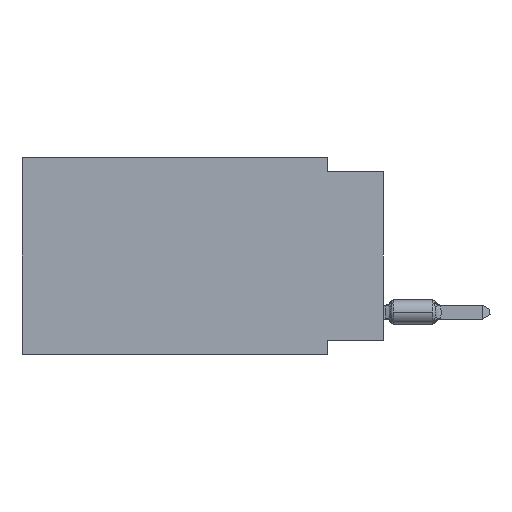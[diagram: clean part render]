
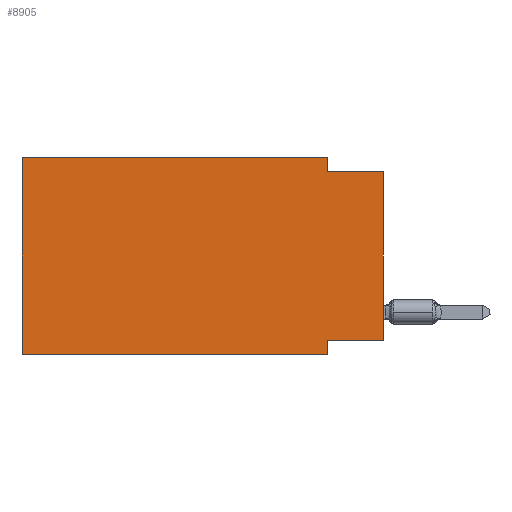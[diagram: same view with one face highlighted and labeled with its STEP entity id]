
A CAD part, left-side view. The second image highlights one B-rep face of the part: STEP entity #8905.
In plain terms, the highlighted planar face has unit normal (-1, 0, 0).
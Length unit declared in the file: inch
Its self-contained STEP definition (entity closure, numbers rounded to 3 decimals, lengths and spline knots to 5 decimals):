
#45 = ORIENTED_EDGE ( 'NONE', *, *, #11545, .F. ) ;
#162 = CARTESIAN_POINT ( 'NONE',  ( 0., 0.645, -0.35 ) ) ;
#1370 = EDGE_CURVE ( 'NONE', #24285, #9462, #19959, .T. ) ;
#2396 = CARTESIAN_POINT ( 'NONE',  ( 0., 0.645, 0. ) ) ;
#3505 = CARTESIAN_POINT ( 'NONE',  ( 0., 0., -0.025 ) ) ;
#4246 = CARTESIAN_POINT ( 'NONE',  ( 0., 0., 0. ) ) ;
#4253 = CARTESIAN_POINT ( 'NONE',  ( 0., 0.1, -0.35 ) ) ;
#4673 = VECTOR ( 'NONE', #25374, 39.37008 ) ;
#6394 = VERTEX_POINT ( 'NONE', #11182 ) ;
#8007 = ORIENTED_EDGE ( 'NONE', *, *, #1370, .T. ) ;
#8520 = LINE ( 'NONE', #3505, #23439 ) ;
#8905 = ADVANCED_FACE ( 'NONE', ( #8964 ), #26022, .F. ) ;
#8964 = FACE_OUTER_BOUND ( 'NONE', #26578, .T. ) ;
#9452 = DIRECTION ( 'NONE',  ( 0., 0., -1. ) ) ;
#9462 = VERTEX_POINT ( 'NONE', #4253 ) ;
#10016 = ORIENTED_EDGE ( 'NONE', *, *, #18518, .T. ) ;
#10137 = VECTOR ( 'NONE', #22067, 39.37008 ) ;
#11182 = CARTESIAN_POINT ( 'NONE',  ( 0., 0., -0.025 ) ) ;
#11545 = EDGE_CURVE ( 'NONE', #32569, #17454, #35048, .T. ) ;
#12277 = AXIS2_PLACEMENT_3D ( 'NONE', #20252, #34721, #31595 ) ;
#13500 = LINE ( 'NONE', #2396, #34774 ) ;
#14606 = ORIENTED_EDGE ( 'NONE', *, *, #29469, .F. ) ;
#15183 = ORIENTED_EDGE ( 'NONE', *, *, #36416, .F. ) ;
#15213 = VERTEX_POINT ( 'NONE', #34568 ) ;
#16543 = CARTESIAN_POINT ( 'NONE',  ( 0., 0.645, -0.35 ) ) ;
#16590 = LINE ( 'NONE', #22883, #17848 ) ;
#17033 = VERTEX_POINT ( 'NONE', #29630 ) ;
#17454 = VERTEX_POINT ( 'NONE', #18063 ) ;
#17838 = ORIENTED_EDGE ( 'NONE', *, *, #32672, .F. ) ;
#17848 = VECTOR ( 'NONE', #36665, 39.37008 ) ;
#18063 = CARTESIAN_POINT ( 'NONE',  ( 0., 0.1, -0.025 ) ) ;
#18518 = EDGE_CURVE ( 'NONE', #17033, #6394, #19054, .T. ) ;
#19054 = LINE ( 'NONE', #4246, #22091 ) ;
#19959 = LINE ( 'NONE', #162, #4673 ) ;
#20252 = CARTESIAN_POINT ( 'NONE',  ( 0., 0.645, 0. ) ) ;
#20347 = DIRECTION ( 'NONE',  ( 0., -1., 0. ) ) ;
#21973 = VECTOR ( 'NONE', #9452, 39.37008 ) ;
#22067 = DIRECTION ( 'NONE',  ( 0., 0., 1. ) ) ;
#22091 = VECTOR ( 'NONE', #29824, 39.37008 ) ;
#22205 = DIRECTION ( 'NONE',  ( 0., -1., 0. ) ) ;
#22883 = CARTESIAN_POINT ( 'NONE',  ( 0., 0., -0.325 ) ) ;
#22989 = VECTOR ( 'NONE', #27749, 39.37008 ) ;
#23093 = EDGE_CURVE ( 'NONE', #15213, #32569, #13500, .T. ) ;
#23439 = VECTOR ( 'NONE', #20347, 39.37008 ) ;
#23898 = CARTESIAN_POINT ( 'NONE',  ( 0., 0.1, 0. ) ) ;
#24285 = VERTEX_POINT ( 'NONE', #16543 ) ;
#24660 = CARTESIAN_POINT ( 'NONE',  ( 0., 0.645, 0. ) ) ;
#25374 = DIRECTION ( 'NONE',  ( 0., -1., 0. ) ) ;
#26022 = PLANE ( 'NONE',  #12277 ) ;
#26578 = EDGE_LOOP ( 'NONE', ( #10016, #17838, #45, #35290, #33995, #8007, #15183, #14606 ) ) ;
#27449 = EDGE_CURVE ( 'NONE', #24285, #15213, #36382, .T. ) ;
#27749 = DIRECTION ( 'NONE',  ( 0., 0., -1. ) ) ;
#28303 = LINE ( 'NONE', #36297, #22989 ) ;
#29469 = EDGE_CURVE ( 'NONE', #17033, #29840, #16590, .T. ) ;
#29630 = CARTESIAN_POINT ( 'NONE',  ( 0., 0., -0.325 ) ) ;
#29824 = DIRECTION ( 'NONE',  ( 0., 0., 1. ) ) ;
#29840 = VERTEX_POINT ( 'NONE', #35145 ) ;
#31595 = DIRECTION ( 'NONE',  ( 0., 0., -1. ) ) ;
#32569 = VERTEX_POINT ( 'NONE', #35982 ) ;
#32672 = EDGE_CURVE ( 'NONE', #17454, #6394, #8520, .T. ) ;
#33995 = ORIENTED_EDGE ( 'NONE', *, *, #27449, .F. ) ;
#34568 = CARTESIAN_POINT ( 'NONE',  ( 0., 0.645, 0. ) ) ;
#34721 = DIRECTION ( 'NONE',  ( 1., 0., 0. ) ) ;
#34774 = VECTOR ( 'NONE', #22205, 39.37008 ) ;
#35048 = LINE ( 'NONE', #23898, #21973 ) ;
#35145 = CARTESIAN_POINT ( 'NONE',  ( 0., 0.1, -0.325 ) ) ;
#35290 = ORIENTED_EDGE ( 'NONE', *, *, #23093, .F. ) ;
#35982 = CARTESIAN_POINT ( 'NONE',  ( 0., 0.1, 0. ) ) ;
#36297 = CARTESIAN_POINT ( 'NONE',  ( 0., 0.1, -0.35 ) ) ;
#36382 = LINE ( 'NONE', #24660, #10137 ) ;
#36416 = EDGE_CURVE ( 'NONE', #29840, #9462, #28303, .T. ) ;
#36665 = DIRECTION ( 'NONE',  ( 0., 1., 0. ) ) ;
